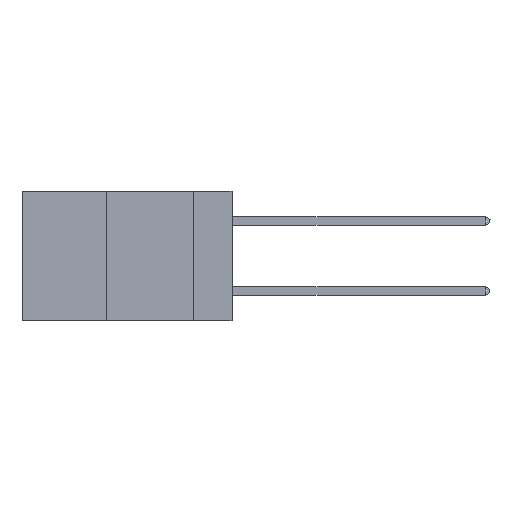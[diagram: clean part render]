
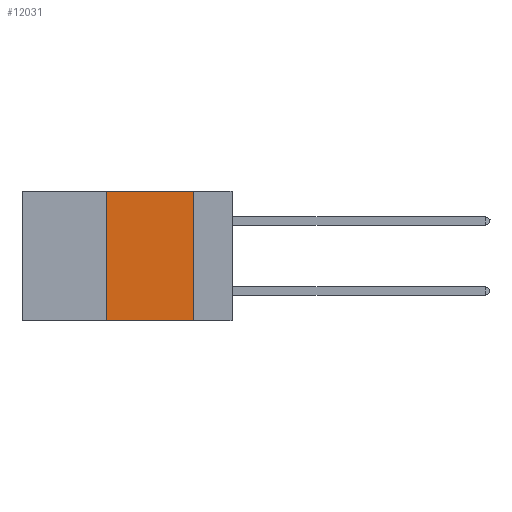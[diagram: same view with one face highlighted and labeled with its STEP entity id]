
A CAD part, left-side view. The second image highlights one B-rep face of the part: STEP entity #12031.
In plain terms, the highlighted planar face has unit normal (-1, 0, 0).
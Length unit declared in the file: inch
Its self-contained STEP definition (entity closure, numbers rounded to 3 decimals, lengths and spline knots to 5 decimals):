
#747 = EDGE_CURVE ( 'NONE', #23999, #27334, #24987, .T. ) ;
#2647 = EDGE_CURVE ( 'NONE', #23999, #24352, #17426, .T. ) ;
#3358 = EDGE_CURVE ( 'NONE', #24352, #22002, #22502, .T. ) ;
#4460 = CARTESIAN_POINT ( 'NONE',  ( 0., 0.6, 0. ) ) ;
#5004 = DIRECTION ( 'NONE',  ( 0., 0., 1. ) ) ;
#6056 = DIRECTION ( 'NONE',  ( 0., -1., 0. ) ) ;
#6350 = ORIENTED_EDGE ( 'NONE', *, *, #747, .T. ) ;
#6735 = VECTOR ( 'NONE', #26926, 39.37008 ) ;
#6963 = EDGE_LOOP ( 'NONE', ( #8506, #11275, #26185, #6350 ) ) ;
#6998 = CARTESIAN_POINT ( 'NONE',  ( 0., 0.11, 0. ) ) ;
#7266 = CARTESIAN_POINT ( 'NONE',  ( 0., 0.36, 0. ) ) ;
#8017 = DIRECTION ( 'NONE',  ( 0., -1., 0. ) ) ;
#8236 = CARTESIAN_POINT ( 'NONE',  ( 0., 0.6, 0. ) ) ;
#8506 = ORIENTED_EDGE ( 'NONE', *, *, #25734, .F. ) ;
#9671 = CARTESIAN_POINT ( 'NONE',  ( 0., 0.11, 0. ) ) ;
#10912 = PLANE ( 'NONE',  #25493 ) ;
#11275 = ORIENTED_EDGE ( 'NONE', *, *, #3358, .F. ) ;
#12031 = ADVANCED_FACE ( 'NONE', ( #15932 ), #10912, .F. ) ;
#12175 = CARTESIAN_POINT ( 'NONE',  ( 0., 0.6, -0.37 ) ) ;
#13055 = DIRECTION ( 'NONE',  ( 1., 0., 0. ) ) ;
#15932 = FACE_OUTER_BOUND ( 'NONE', #6963, .T. ) ;
#17426 = LINE ( 'NONE', #7266, #23848 ) ;
#19123 = VECTOR ( 'NONE', #6056, 39.37008 ) ;
#19597 = CARTESIAN_POINT ( 'NONE',  ( 0., 0.36, 0. ) ) ;
#21269 = VECTOR ( 'NONE', #8017, 39.37008 ) ;
#22002 = VERTEX_POINT ( 'NONE', #6998 ) ;
#22502 = LINE ( 'NONE', #8236, #19123 ) ;
#23674 = DIRECTION ( 'NONE',  ( 0., 0., -1. ) ) ;
#23758 = CARTESIAN_POINT ( 'NONE',  ( 0., 0.11, -0.37 ) ) ;
#23848 = VECTOR ( 'NONE', #5004, 39.37008 ) ;
#23999 = VERTEX_POINT ( 'NONE', #27048 ) ;
#24352 = VERTEX_POINT ( 'NONE', #19597 ) ;
#24923 = LINE ( 'NONE', #9671, #6735 ) ;
#24987 = LINE ( 'NONE', #12175, #21269 ) ;
#25493 = AXIS2_PLACEMENT_3D ( 'NONE', #4460, #13055, #23674 ) ;
#25734 = EDGE_CURVE ( 'NONE', #22002, #27334, #24923, .T. ) ;
#26185 = ORIENTED_EDGE ( 'NONE', *, *, #2647, .F. ) ;
#26926 = DIRECTION ( 'NONE',  ( 0., 0., -1. ) ) ;
#27048 = CARTESIAN_POINT ( 'NONE',  ( 0., 0.36, -0.37 ) ) ;
#27334 = VERTEX_POINT ( 'NONE', #23758 ) ;
